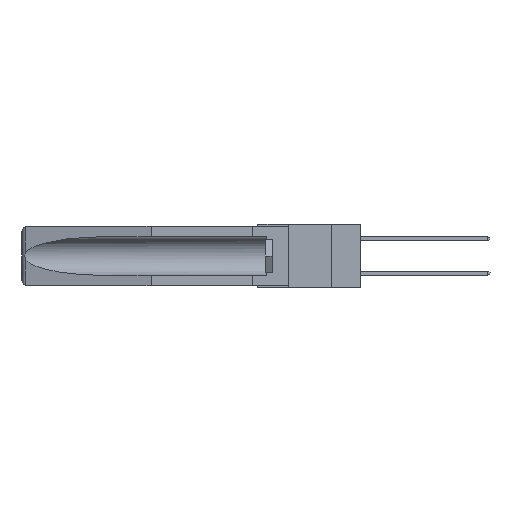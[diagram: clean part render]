
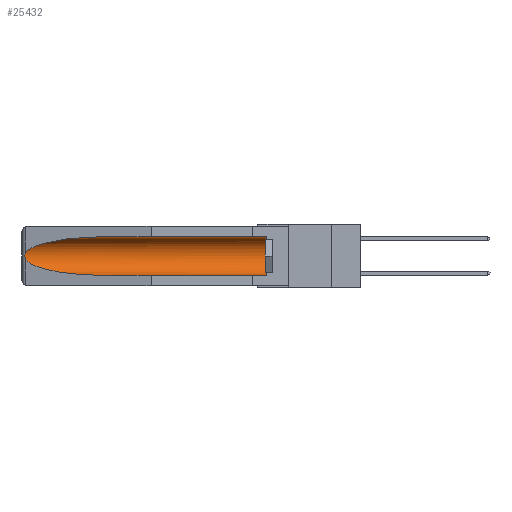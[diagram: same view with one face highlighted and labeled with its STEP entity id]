
A CAD part, left-side view. The second image highlights one B-rep face of the part: STEP entity #25432.
In plain terms, the highlighted cylindrical face has radius 2.857 mm (diameter 5.715 mm), a partial arc.
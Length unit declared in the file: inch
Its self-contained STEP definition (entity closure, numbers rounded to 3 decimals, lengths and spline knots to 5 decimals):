
#597 = CARTESIAN_POINT ( 'NONE',  ( 0.26537, 1.52718, -0.19328 ) ) ;
#695 = EDGE_LOOP ( 'NONE', ( #16646, #1110, #24684, #3274, #11255, #24911 ) ) ;
#1110 = ORIENTED_EDGE ( 'NONE', *, *, #7423, .T. ) ;
#1438 = AXIS2_PLACEMENT_3D ( 'NONE', #22356, #8666, #22254 ) ;
#1682 = CARTESIAN_POINT ( 'NONE',  ( 0.25451, 1.48313, -0.09465 ) ) ;
#1971 = CARTESIAN_POINT ( 'NONE',  ( 0.155, 1.07973, -0.059 ) ) ;
#2884 = VERTEX_POINT ( 'NONE', #3260 ) ;
#3125 = CARTESIAN_POINT ( 'NONE',  ( 0.25451, 1.48313, -0.24835 ) ) ;
#3260 = CARTESIAN_POINT ( 'NONE',  ( 0.26537, 1.52718, -0.14972 ) ) ;
#3274 = ORIENTED_EDGE ( 'NONE', *, *, #5332, .F. ) ;
#4997 = CARTESIAN_POINT ( 'NONE',  ( 0.155, -0.30754, -0.059 ) ) ;
#5202 =( BOUNDED_CURVE ( )  B_SPLINE_CURVE ( 3, ( #597, #3125, #10195, #28161 ),
 .UNSPECIFIED., .F., .F. ) 
 B_SPLINE_CURVE_WITH_KNOTS ( ( 4, 4 ),
 ( 0.1948, 1.5708 ),
 .UNSPECIFIED. ) 
 CURVE ( )  GEOMETRIC_REPRESENTATION_ITEM ( )  RATIONAL_B_SPLINE_CURVE ( ( 1., 0.848, 0.848, 1. ) ) 
 REPRESENTATION_ITEM ( '' )  );
#5233 = CARTESIAN_POINT ( 'NONE',  ( 0.2673, 1.53269, -0.17917 ) ) ;
#5332 = EDGE_CURVE ( 'NONE', #12861, #25028, #10767, .T. ) ;
#7423 = EDGE_CURVE ( 'NONE', #2884, #28679, #21136, .T. ) ;
#7549 = CARTESIAN_POINT ( 'NONE',  ( 0.26597, 1.52961, -0.15275 ) ) ;
#8239 = CARTESIAN_POINT ( 'NONE',  ( 0.155, -0.30754, -0.284 ) ) ;
#8311 =( BOUNDED_CURVE ( )  B_SPLINE_CURVE ( 3, ( #24036, #29484, #1682, #15682 ),
 .UNSPECIFIED., .F., .F. ) 
 B_SPLINE_CURVE_WITH_KNOTS ( ( 4, 4 ),
 ( 4.71239, 6.08839 ),
 .UNSPECIFIED. ) 
 CURVE ( )  GEOMETRIC_REPRESENTATION_ITEM ( )  RATIONAL_B_SPLINE_CURVE ( ( 1., 0.848, 0.848, 1. ) ) 
 REPRESENTATION_ITEM ( '' )  );
#8666 = DIRECTION ( 'NONE',  ( 0., 1., 0. ) ) ;
#10195 = CARTESIAN_POINT ( 'NONE',  ( 0.21114, 1.30732, -0.284 ) ) ;
#10767 = LINE ( 'NONE', #8239, #26573 ) ;
#10778 = CARTESIAN_POINT ( 'NONE',  ( 0.155, 1.07973, -0.284 ) ) ;
#11255 = ORIENTED_EDGE ( 'NONE', *, *, #17816, .T. ) ;
#11520 = DIRECTION ( 'NONE',  ( 0., 0., 1. ) ) ;
#11551 = CARTESIAN_POINT ( 'NONE',  ( 0.155, 0.126, -0.059 ) ) ;
#11951 = CARTESIAN_POINT ( 'NONE',  ( 0.26654, 1.53092, -0.15636 ) ) ;
#12459 = EDGE_CURVE ( 'NONE', #28679, #25028, #5202, .T. ) ;
#12861 = VERTEX_POINT ( 'NONE', #20732 ) ;
#13049 = CIRCLE ( 'NONE', #17699, 0.1125 ) ;
#13839 = VECTOR ( 'NONE', #27876, 39.37008 ) ;
#14248 = CARTESIAN_POINT ( 'NONE',  ( 0.26537, 1.52718, -0.14972 ) ) ;
#14443 = CARTESIAN_POINT ( 'NONE',  ( 0.2675, 1.53308, -0.16763 ) ) ;
#15682 = CARTESIAN_POINT ( 'NONE',  ( 0.26537, 1.52718, -0.14972 ) ) ;
#16216 = CARTESIAN_POINT ( 'NONE',  ( 0.26597, 1.5296, -0.19026 ) ) ;
#16417 = CARTESIAN_POINT ( 'NONE',  ( 0.155, 0.126, -0.1715 ) ) ;
#16561 = CARTESIAN_POINT ( 'NONE',  ( 0.26537, 1.52718, -0.19328 ) ) ;
#16646 = ORIENTED_EDGE ( 'NONE', *, *, #19442, .T. ) ;
#17699 = AXIS2_PLACEMENT_3D ( 'NONE', #16417, #20708, #11520 ) ;
#17816 = EDGE_CURVE ( 'NONE', #12861, #20261, #13049, .T. ) ;
#18490 = CARTESIAN_POINT ( 'NONE',  ( 0.26537, 1.52718, -0.19328 ) ) ;
#18800 = FACE_OUTER_BOUND ( 'NONE', #695, .T. ) ;
#18896 = CARTESIAN_POINT ( 'NONE',  ( 0.2675, 1.53308, -0.17534 ) ) ;
#19442 = EDGE_CURVE ( 'NONE', #24348, #2884, #8311, .T. ) ;
#20261 = VERTEX_POINT ( 'NONE', #11551 ) ;
#20708 = DIRECTION ( 'NONE',  ( 0., -1., 0. ) ) ;
#20732 = CARTESIAN_POINT ( 'NONE',  ( 0.155, 0.126, -0.284 ) ) ;
#21118 = CARTESIAN_POINT ( 'NONE',  ( 0.2673, 1.5327, -0.16383 ) ) ;
#21136 = B_SPLINE_CURVE_WITH_KNOTS ( 'NONE', 3,
 ( #14248, #7549, #11951, #21118, #14443, #18896, #5233, #25887, #16216, #18490 ),
 .UNSPECIFIED., .F., .F.,
 ( 4, 2, 2, 2, 4 ),
 ( 0., 0.00029, 0.00058, 0.00087, 0.00117 ),
 .UNSPECIFIED. ) ;
#22254 = DIRECTION ( 'NONE',  ( 0., 0., 1. ) ) ;
#22356 = CARTESIAN_POINT ( 'NONE',  ( 0.155, -0.30754, -0.1715 ) ) ;
#24036 = CARTESIAN_POINT ( 'NONE',  ( 0.155, 1.07973, -0.059 ) ) ;
#24348 = VERTEX_POINT ( 'NONE', #1971 ) ;
#24548 = CYLINDRICAL_SURFACE ( 'NONE', #1438, 0.1125 ) ;
#24684 = ORIENTED_EDGE ( 'NONE', *, *, #12459, .T. ) ;
#24911 = ORIENTED_EDGE ( 'NONE', *, *, #25196, .T. ) ;
#25028 = VERTEX_POINT ( 'NONE', #10778 ) ;
#25196 = EDGE_CURVE ( 'NONE', #20261, #24348, #26078, .T. ) ;
#25432 = ADVANCED_FACE ( 'NONE', ( #18800 ), #24548, .F. ) ;
#25887 = CARTESIAN_POINT ( 'NONE',  ( 0.26655, 1.53094, -0.18657 ) ) ;
#26078 = LINE ( 'NONE', #4997, #13839 ) ;
#26573 = VECTOR ( 'NONE', #28912, 39.37008 ) ;
#27876 = DIRECTION ( 'NONE',  ( 0., 1., 0. ) ) ;
#28161 = CARTESIAN_POINT ( 'NONE',  ( 0.155, 1.07973, -0.284 ) ) ;
#28679 = VERTEX_POINT ( 'NONE', #16561 ) ;
#28912 = DIRECTION ( 'NONE',  ( 0., 1., 0. ) ) ;
#29484 = CARTESIAN_POINT ( 'NONE',  ( 0.21114, 1.30732, -0.059 ) ) ;
